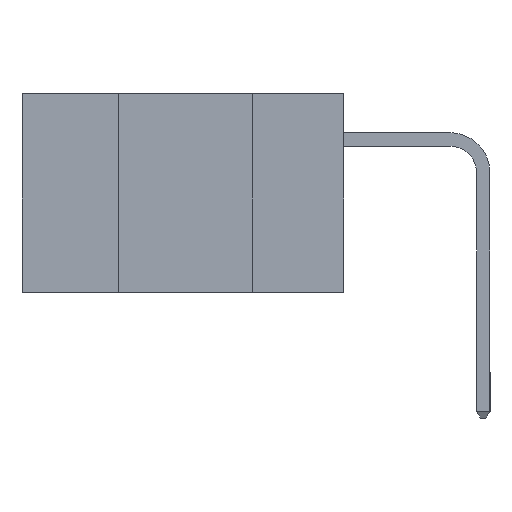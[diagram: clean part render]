
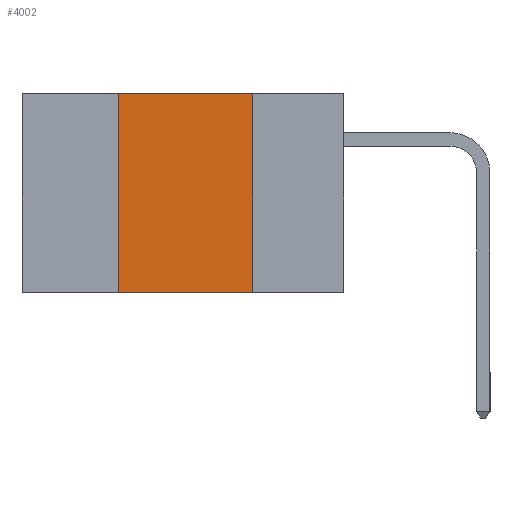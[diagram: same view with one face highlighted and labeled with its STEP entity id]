
A CAD part, left-side view. The second image highlights one B-rep face of the part: STEP entity #4002.
In plain terms, the highlighted planar face has unit normal (-1, 0, 0).
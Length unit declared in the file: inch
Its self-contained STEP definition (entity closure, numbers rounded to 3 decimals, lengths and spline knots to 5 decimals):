
#1 = VERTEX_POINT ( 'NONE', #23999 ) ;
#381 = CARTESIAN_POINT ( 'NONE',  ( 0., 0.6, 0. ) ) ;
#583 = CARTESIAN_POINT ( 'NONE',  ( 0., 0.6, -0.37 ) ) ;
#1489 = ORIENTED_EDGE ( 'NONE', *, *, #24273, .F. ) ;
#3389 = ORIENTED_EDGE ( 'NONE', *, *, #4431, .T. ) ;
#4002 = ADVANCED_FACE ( 'NONE', ( #13034 ), #8135, .F. ) ;
#4431 = EDGE_CURVE ( 'NONE', #1, #17896, #12728, .T. ) ;
#5362 = VERTEX_POINT ( 'NONE', #17744 ) ;
#6335 = DIRECTION ( 'NONE',  ( 0., -1., 0. ) ) ;
#6493 = VECTOR ( 'NONE', #25050, 39.37008 ) ;
#6619 = DIRECTION ( 'NONE',  ( 0., -1., 0. ) ) ;
#8135 = PLANE ( 'NONE',  #8627 ) ;
#8627 = AXIS2_PLACEMENT_3D ( 'NONE', #381, #14058, #18159 ) ;
#10465 = CARTESIAN_POINT ( 'NONE',  ( 0., 0.6, 0. ) ) ;
#11243 = VERTEX_POINT ( 'NONE', #21465 ) ;
#11709 = LINE ( 'NONE', #12053, #6493 ) ;
#12053 = CARTESIAN_POINT ( 'NONE',  ( 0., 0.17, 0. ) ) ;
#12239 = CARTESIAN_POINT ( 'NONE',  ( 0., 0.17, -0.37 ) ) ;
#12728 = LINE ( 'NONE', #583, #22482 ) ;
#13034 = FACE_OUTER_BOUND ( 'NONE', #19866, .T. ) ;
#13441 = VECTOR ( 'NONE', #6335, 39.37008 ) ;
#13954 = ORIENTED_EDGE ( 'NONE', *, *, #16994, .F. ) ;
#14058 = DIRECTION ( 'NONE',  ( 1., 0., 0. ) ) ;
#15226 = ORIENTED_EDGE ( 'NONE', *, *, #23786, .F. ) ;
#15429 = DIRECTION ( 'NONE',  ( 0., 0., 1. ) ) ;
#16994 = EDGE_CURVE ( 'NONE', #5362, #17896, #11709, .T. ) ;
#17744 = CARTESIAN_POINT ( 'NONE',  ( 0., 0.17, 0. ) ) ;
#17896 = VERTEX_POINT ( 'NONE', #12239 ) ;
#18159 = DIRECTION ( 'NONE',  ( 0., 0., -1. ) ) ;
#18334 = VECTOR ( 'NONE', #15429, 39.37008 ) ;
#19823 = LINE ( 'NONE', #10465, #13441 ) ;
#19866 = EDGE_LOOP ( 'NONE', ( #13954, #15226, #1489, #3389 ) ) ;
#21227 = CARTESIAN_POINT ( 'NONE',  ( 0., 0.42, 0. ) ) ;
#21465 = CARTESIAN_POINT ( 'NONE',  ( 0., 0.42, 0. ) ) ;
#22482 = VECTOR ( 'NONE', #6619, 39.37008 ) ;
#22920 = LINE ( 'NONE', #21227, #18334 ) ;
#23786 = EDGE_CURVE ( 'NONE', #11243, #5362, #19823, .T. ) ;
#23999 = CARTESIAN_POINT ( 'NONE',  ( 0., 0.42, -0.37 ) ) ;
#24273 = EDGE_CURVE ( 'NONE', #1, #11243, #22920, .T. ) ;
#25050 = DIRECTION ( 'NONE',  ( 0., 0., -1. ) ) ;
